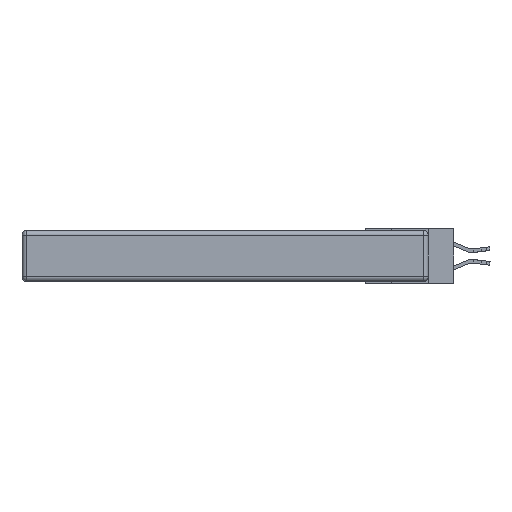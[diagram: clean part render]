
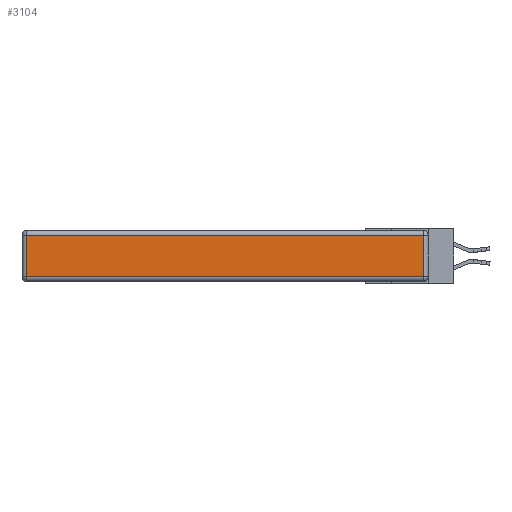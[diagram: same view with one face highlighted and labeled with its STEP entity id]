
A CAD part, left-side view. The second image highlights one B-rep face of the part: STEP entity #3104.
In plain terms, the highlighted planar face has unit normal (-1, 0, 0).
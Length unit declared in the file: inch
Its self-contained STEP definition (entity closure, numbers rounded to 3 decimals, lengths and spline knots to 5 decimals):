
#606 = VECTOR ( 'NONE', #10271, 39.37008 ) ;
#2294 = CARTESIAN_POINT ( 'NONE',  ( 0., 0., -0.343 ) ) ;
#2586 = CARTESIAN_POINT ( 'NONE',  ( 0., 2.72, -0.313 ) ) ;
#3104 = ADVANCED_FACE ( 'NONE', ( #12388 ), #3467, .T. ) ;
#3199 = CARTESIAN_POINT ( 'NONE',  ( 0., 2.75, -0.03 ) ) ;
#3413 = DIRECTION ( 'NONE',  ( -1., 0., 0. ) ) ;
#3467 = PLANE ( 'NONE',  #5980 ) ;
#3544 = LINE ( 'NONE', #5529, #12450 ) ;
#4099 = CARTESIAN_POINT ( 'NONE',  ( 0., 2.72, -0.03 ) ) ;
#4248 = DIRECTION ( 'NONE',  ( 0., 0., -1. ) ) ;
#4298 = LINE ( 'NONE', #3199, #5688 ) ;
#4972 = LINE ( 'NONE', #8036, #606 ) ;
#4990 = EDGE_LOOP ( 'NONE', ( #13270, #13228, #8436, #6338 ) ) ;
#5085 = VERTEX_POINT ( 'NONE', #5445 ) ;
#5260 = EDGE_CURVE ( 'NONE', #10635, #5085, #3544, .T. ) ;
#5380 = DIRECTION ( 'NONE',  ( 0., 1., 0. ) ) ;
#5436 = LINE ( 'NONE', #14383, #5783 ) ;
#5445 = CARTESIAN_POINT ( 'NONE',  ( 0., 0.03, -0.03 ) ) ;
#5529 = CARTESIAN_POINT ( 'NONE',  ( 0., 0.03, -0.343 ) ) ;
#5607 = CARTESIAN_POINT ( 'NONE',  ( 0., 0.03, -0.313 ) ) ;
#5688 = VECTOR ( 'NONE', #5380, 39.37008 ) ;
#5783 = VECTOR ( 'NONE', #4248, 39.37008 ) ;
#5980 = AXIS2_PLACEMENT_3D ( 'NONE', #2294, #3413, #13544 ) ;
#6338 = ORIENTED_EDGE ( 'NONE', *, *, #12085, .T. ) ;
#8036 = CARTESIAN_POINT ( 'NONE',  ( 0., 0., -0.313 ) ) ;
#8224 = VERTEX_POINT ( 'NONE', #4099 ) ;
#8436 = ORIENTED_EDGE ( 'NONE', *, *, #8991, .T. ) ;
#8915 = DIRECTION ( 'NONE',  ( 0., 0., 1. ) ) ;
#8991 = EDGE_CURVE ( 'NONE', #5085, #8224, #4298, .T. ) ;
#10271 = DIRECTION ( 'NONE',  ( 0., -1., 0. ) ) ;
#10635 = VERTEX_POINT ( 'NONE', #5607 ) ;
#10779 = EDGE_CURVE ( 'NONE', #12425, #10635, #4972, .T. ) ;
#12085 = EDGE_CURVE ( 'NONE', #8224, #12425, #5436, .T. ) ;
#12388 = FACE_OUTER_BOUND ( 'NONE', #4990, .T. ) ;
#12425 = VERTEX_POINT ( 'NONE', #2586 ) ;
#12450 = VECTOR ( 'NONE', #8915, 39.37008 ) ;
#13228 = ORIENTED_EDGE ( 'NONE', *, *, #5260, .T. ) ;
#13270 = ORIENTED_EDGE ( 'NONE', *, *, #10779, .T. ) ;
#13544 = DIRECTION ( 'NONE',  ( 0., 0., 1. ) ) ;
#14383 = CARTESIAN_POINT ( 'NONE',  ( 0., 2.72, -0.343 ) ) ;
